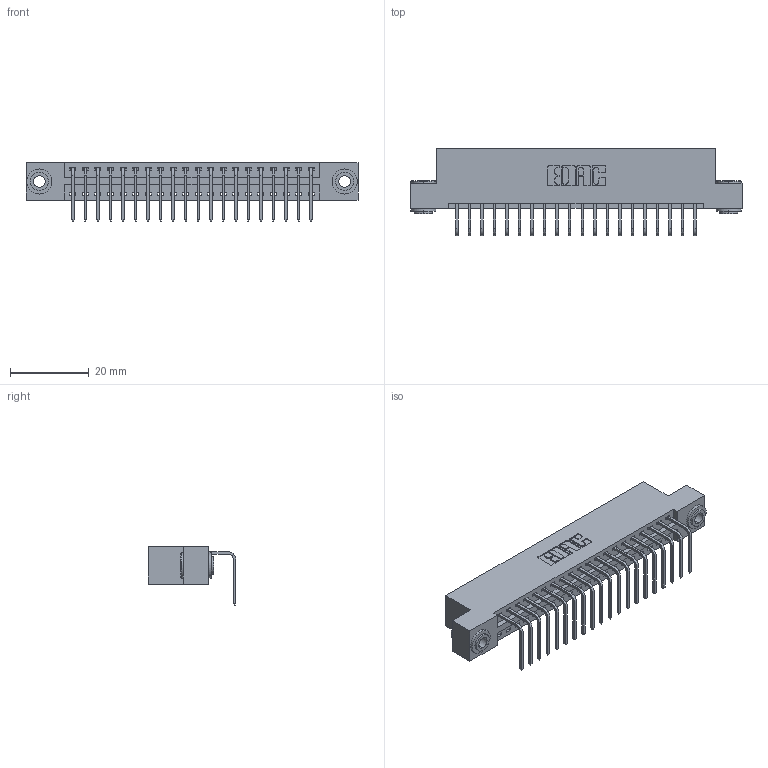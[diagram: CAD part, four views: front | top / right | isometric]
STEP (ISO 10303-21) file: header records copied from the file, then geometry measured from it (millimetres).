
FILE_DESCRIPTION (( 'STEP AP203' ), '1' );
FILE_NAME ('346-020-558-103.STEP', '2022-05-05T17:05:33', ( '' ), ( '' ), 'SwSTEP 2.0', 'SolidWorks 2020', '' );
FILE_SCHEMA (( 'CONFIG_CONTROL_DESIGN' ));
Length unit declared in the file: inch
Products named in the file (4): 345-250-002_345-250-002-102; 345-292-001_558 Tail - 2; 346 Part_Flush Mounting Lugs - 0.156 Dia-TH; 346-020-558-103
Assembly tree (23 placements, depth 2):
  346-020-558-103
    346 Part_Flush Mounting Lugs - 0.156 Dia-TH
    345-292-001_558 Tail - 2  x20
    345-250-002_345-250-002-102  x2
Bounding box: 84.07 x 22.16 x 14.73 mm (x, y, z)
Volume: 7964.1 mm3; surface area: 10365.7 mm2
Topology: 23 solids, 23 shells, 1374 faces, 4081 edges, 2690 vertices
Faces by surface type: plane 940, cylinder 426, cone 8
Entity records: 16524 total; most frequent: CARTESIAN_POINT 2821, ORIENTED_EDGE 2766, DIRECTION 2545, EDGE_CURVE 1383, LINE 1147, VECTOR 1147, VERTEX_POINT 918, AXIS2_PLACEMENT_3D 699
